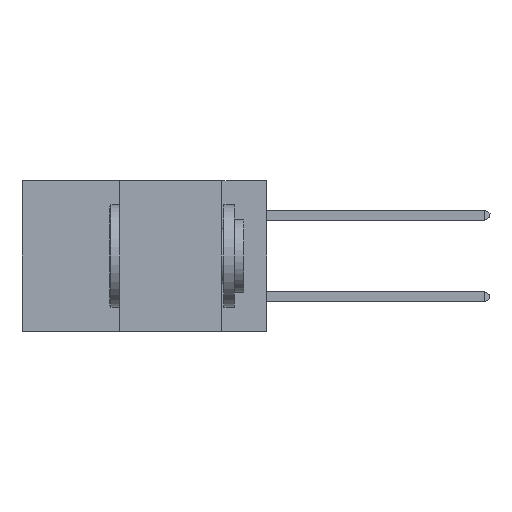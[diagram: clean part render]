
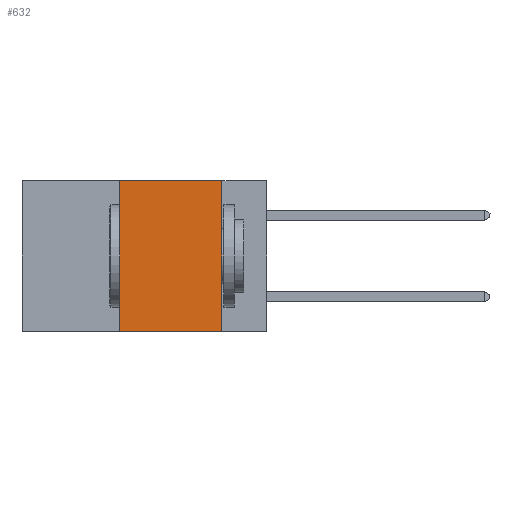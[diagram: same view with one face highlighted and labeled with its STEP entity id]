
A CAD part, left-side view. The second image highlights one B-rep face of the part: STEP entity #632.
In plain terms, the highlighted planar face has unit normal (-1, 0, 0).
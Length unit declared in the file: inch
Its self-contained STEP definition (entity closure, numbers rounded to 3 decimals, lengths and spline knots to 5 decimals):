
#632 = ADVANCED_FACE ( 'NONE', ( #8432 ), #3442, .F. ) ;
#1382 = DIRECTION ( 'NONE',  ( 0., 0., 1. ) ) ;
#1755 = VERTEX_POINT ( 'NONE', #3249 ) ;
#2282 = CARTESIAN_POINT ( 'NONE',  ( 0., 0.36, 0. ) ) ;
#3078 = VECTOR ( 'NONE', #6255, 39.37008 ) ;
#3249 = CARTESIAN_POINT ( 'NONE',  ( 0., 0.11, -0.37 ) ) ;
#3442 = PLANE ( 'NONE',  #6777 ) ;
#3778 = EDGE_CURVE ( 'NONE', #8812, #1755, #8207, .T. ) ;
#3781 = EDGE_CURVE ( 'NONE', #6388, #1755, #5677, .T. ) ;
#4137 = EDGE_CURVE ( 'NONE', #6388, #10555, #5384, .T. ) ;
#4257 = ORIENTED_EDGE ( 'NONE', *, *, #3778, .F. ) ;
#4673 = ORIENTED_EDGE ( 'NONE', *, *, #7886, .F. ) ;
#4815 = CARTESIAN_POINT ( 'NONE',  ( 0., 0.11, 0. ) ) ;
#5384 = LINE ( 'NONE', #2282, #12316 ) ;
#5677 = LINE ( 'NONE', #6772, #10333 ) ;
#6050 = DIRECTION ( 'NONE',  ( 0., -1., 0. ) ) ;
#6255 = DIRECTION ( 'NONE',  ( 0., 0., -1. ) ) ;
#6388 = VERTEX_POINT ( 'NONE', #8447 ) ;
#6651 = CARTESIAN_POINT ( 'NONE',  ( 0., 0.11, 0. ) ) ;
#6772 = CARTESIAN_POINT ( 'NONE',  ( 0., 0.6, -0.37 ) ) ;
#6777 = AXIS2_PLACEMENT_3D ( 'NONE', #10598, #12278, #11407 ) ;
#7356 = DIRECTION ( 'NONE',  ( 0., -1., 0. ) ) ;
#7886 = EDGE_CURVE ( 'NONE', #10555, #8812, #11809, .T. ) ;
#8207 = LINE ( 'NONE', #6651, #3078 ) ;
#8432 = FACE_OUTER_BOUND ( 'NONE', #9812, .T. ) ;
#8435 = CARTESIAN_POINT ( 'NONE',  ( 0., 0.36, 0. ) ) ;
#8447 = CARTESIAN_POINT ( 'NONE',  ( 0., 0.36, -0.37 ) ) ;
#8812 = VERTEX_POINT ( 'NONE', #4815 ) ;
#9415 = ORIENTED_EDGE ( 'NONE', *, *, #3781, .T. ) ;
#9528 = VECTOR ( 'NONE', #7356, 39.37008 ) ;
#9812 = EDGE_LOOP ( 'NONE', ( #4257, #4673, #11706, #9415 ) ) ;
#10333 = VECTOR ( 'NONE', #6050, 39.37008 ) ;
#10555 = VERTEX_POINT ( 'NONE', #8435 ) ;
#10598 = CARTESIAN_POINT ( 'NONE',  ( 0., 0.6, 0. ) ) ;
#11407 = DIRECTION ( 'NONE',  ( 0., 0., -1. ) ) ;
#11706 = ORIENTED_EDGE ( 'NONE', *, *, #4137, .F. ) ;
#11788 = CARTESIAN_POINT ( 'NONE',  ( 0., 0.6, 0. ) ) ;
#11809 = LINE ( 'NONE', #11788, #9528 ) ;
#12278 = DIRECTION ( 'NONE',  ( 1., 0., 0. ) ) ;
#12316 = VECTOR ( 'NONE', #1382, 39.37008 ) ;
